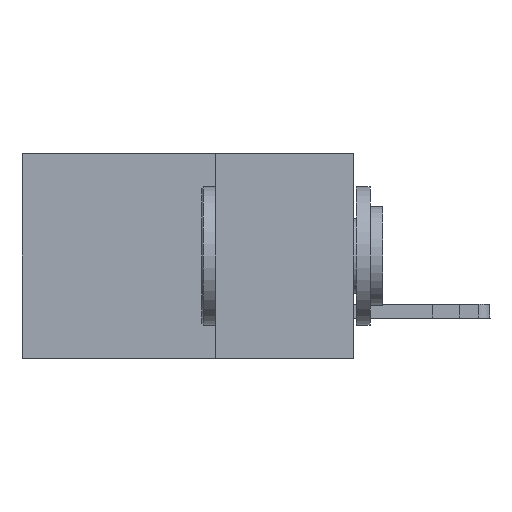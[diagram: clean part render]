
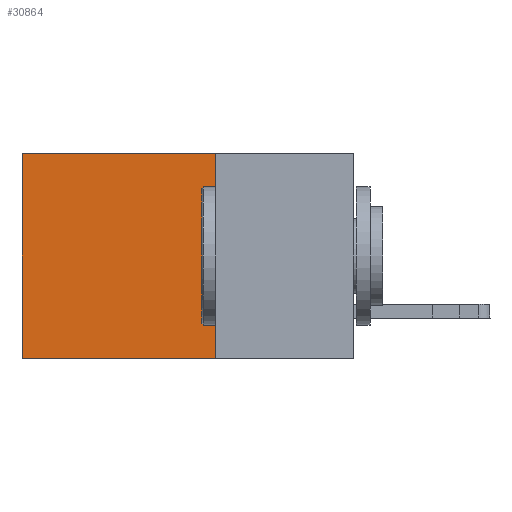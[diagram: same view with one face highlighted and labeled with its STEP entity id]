
A CAD part, left-side view. The second image highlights one B-rep face of the part: STEP entity #30864.
In plain terms, the highlighted planar face has unit normal (-1, 0, 0).
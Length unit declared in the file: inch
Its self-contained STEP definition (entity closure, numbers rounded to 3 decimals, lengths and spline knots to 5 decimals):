
#15 = VERTEX_POINT ( 'NONE', #20705 ) ;
#257 = EDGE_CURVE ( 'NONE', #15, #22873, #16020, .T. ) ;
#935 = AXIS2_PLACEMENT_3D ( 'NONE', #18203, #15704, #20617 ) ;
#1887 = ORIENTED_EDGE ( 'NONE', *, *, #257, .T. ) ;
#2157 = VECTOR ( 'NONE', #6653, 39.37008 ) ;
#2859 = EDGE_CURVE ( 'NONE', #10927, #8488, #28827, .T. ) ;
#3816 = ORIENTED_EDGE ( 'NONE', *, *, #26536, .T. ) ;
#6653 = DIRECTION ( 'NONE',  ( 0., 1., 0. ) ) ;
#7971 = CARTESIAN_POINT ( 'NONE',  ( 0.2875, 0.6, -0.37 ) ) ;
#8488 = VERTEX_POINT ( 'NONE', #7971 ) ;
#10092 = CARTESIAN_POINT ( 'NONE',  ( 0.2875, 0.6, 0. ) ) ;
#10375 = FACE_OUTER_BOUND ( 'NONE', #21463, .T. ) ;
#10927 = VERTEX_POINT ( 'NONE', #30400 ) ;
#12151 = VECTOR ( 'NONE', #15098, 39.37008 ) ;
#12791 = ORIENTED_EDGE ( 'NONE', *, *, #30889, .F. ) ;
#13274 = CARTESIAN_POINT ( 'NONE',  ( 0.2875, 0.25, 0. ) ) ;
#13424 = PLANE ( 'NONE',  #935 ) ;
#13722 = LINE ( 'NONE', #14012, #15218 ) ;
#14012 = CARTESIAN_POINT ( 'NONE',  ( 0.2875, 0.25, 0. ) ) ;
#15098 = DIRECTION ( 'NONE',  ( 0., 0., -1. ) ) ;
#15218 = VECTOR ( 'NONE', #23560, 39.37008 ) ;
#15704 = DIRECTION ( 'NONE',  ( 1., 0., 0. ) ) ;
#16020 = LINE ( 'NONE', #13274, #2157 ) ;
#18203 = CARTESIAN_POINT ( 'NONE',  ( 0.2875, 0.25, 0. ) ) ;
#20617 = DIRECTION ( 'NONE',  ( 0., 0., -1. ) ) ;
#20705 = CARTESIAN_POINT ( 'NONE',  ( 0.2875, 0.25, 0. ) ) ;
#21262 = CARTESIAN_POINT ( 'NONE',  ( 0.2875, 0.6, 0. ) ) ;
#21463 = EDGE_LOOP ( 'NONE', ( #3816, #26576, #12791, #1887 ) ) ;
#22155 = VECTOR ( 'NONE', #24365, 39.37008 ) ;
#22873 = VERTEX_POINT ( 'NONE', #21262 ) ;
#23319 = LINE ( 'NONE', #10092, #12151 ) ;
#23560 = DIRECTION ( 'NONE',  ( 0., 0., -1. ) ) ;
#24365 = DIRECTION ( 'NONE',  ( 0., 1., 0. ) ) ;
#26536 = EDGE_CURVE ( 'NONE', #22873, #8488, #23319, .T. ) ;
#26576 = ORIENTED_EDGE ( 'NONE', *, *, #2859, .F. ) ;
#28827 = LINE ( 'NONE', #28968, #22155 ) ;
#28968 = CARTESIAN_POINT ( 'NONE',  ( 0.2875, 0.25, -0.37 ) ) ;
#30400 = CARTESIAN_POINT ( 'NONE',  ( 0.2875, 0.25, -0.37 ) ) ;
#30864 = ADVANCED_FACE ( 'NONE', ( #10375 ), #13424, .F. ) ;
#30889 = EDGE_CURVE ( 'NONE', #15, #10927, #13722, .T. ) ;
